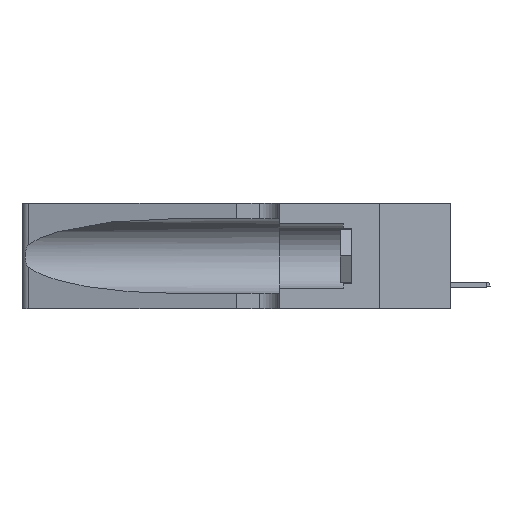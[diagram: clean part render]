
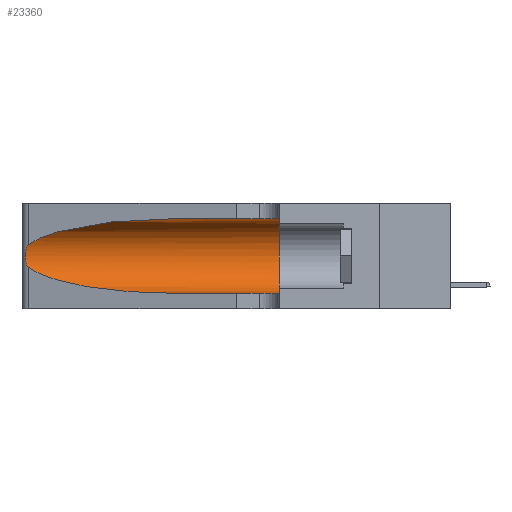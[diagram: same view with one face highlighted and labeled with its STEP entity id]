
A CAD part, left-side view. The second image highlights one B-rep face of the part: STEP entity #23360.
In plain terms, the highlighted cylindrical face has radius 3.308 mm (diameter 6.617 mm), a partial arc.
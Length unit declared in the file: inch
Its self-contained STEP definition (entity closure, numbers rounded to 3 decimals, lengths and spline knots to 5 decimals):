
#435 = ORIENTED_EDGE ( 'NONE', *, *, #18205, .T. ) ;
#545 = VERTEX_POINT ( 'NONE', #1530 ) ;
#792 = VERTEX_POINT ( 'NONE', #42409 ) ;
#1530 = CARTESIAN_POINT ( 'NONE',  ( 0.25487, 1.22718, 0.14631 ) ) ;
#2758 = VERTEX_POINT ( 'NONE', #30562 ) ;
#3268 = ORIENTED_EDGE ( 'NONE', *, *, #11400, .F. ) ;
#3404 = CARTESIAN_POINT ( 'NONE',  ( 0.25555, 1.22994, 0.2215 ) ) ;
#5291 =( BOUNDED_CURVE ( )  B_SPLINE_CURVE ( 3, ( #20249, #23532, #7633, #46288 ),
 .UNSPECIFIED., .F., .F. ) 
 B_SPLINE_CURVE_WITH_KNOTS ( ( 4, 4 ),
 ( 1.5708, 2.84003 ),
 .UNSPECIFIED. ) 
 CURVE ( )  GEOMETRIC_REPRESENTATION_ITEM ( )  RATIONAL_B_SPLINE_CURVE ( ( 1., 0.87, 0.87, 1. ) ) 
 REPRESENTATION_ITEM ( '' )  );
#5547 = DIRECTION ( 'NONE',  ( 0., -1., 0. ) ) ;
#6054 = LINE ( 'NONE', #32336, #23527 ) ;
#6379 = CARTESIAN_POINT ( 'NONE',  ( 0.2373, 1.15595, 0.08982 ) ) ;
#7177 = CARTESIAN_POINT ( 'NONE',  ( 0.25787, 1.23484, 0.2124 ) ) ;
#7300 = DIRECTION ( 'NONE',  ( 0., 1., 0. ) ) ;
#7633 = CARTESIAN_POINT ( 'NONE',  ( 0.2373, 1.15595, 0.28018 ) ) ;
#9476 = AXIS2_PLACEMENT_3D ( 'NONE', #9518, #18070, #14035 ) ;
#9518 = CARTESIAN_POINT ( 'NONE',  ( 0.1305, 1.61858, 0.185 ) ) ;
#10172 = ORIENTED_EDGE ( 'NONE', *, *, #28903, .F. ) ;
#10822 = B_SPLINE_CURVE_WITH_KNOTS ( 'NONE', 3,
 ( #15258, #3404, #15509, #7177, #14499, #22316, #26127, #14998, #33982, #49378, #14746, #18793, #19301, #22567 ),
 .UNSPECIFIED., .F., .F.,
 ( 4, 2, 2, 2, 2, 2, 4 ),
 ( 0., 0.00027, 0.00053, 0.00107, 0.0016, 0.00187, 0.00214 ),
 .UNSPECIFIED. ) ;
#11400 = EDGE_CURVE ( 'NONE', #2758, #25137, #27996, .T. ) ;
#13346 = EDGE_CURVE ( 'NONE', #792, #545, #10822, .T. ) ;
#13796 = CYLINDRICAL_SURFACE ( 'NONE', #9476, 0.13025 ) ;
#14035 = DIRECTION ( 'NONE',  ( 0., 0., -1. ) ) ;
#14499 = CARTESIAN_POINT ( 'NONE',  ( 0.25854, 1.2359, 0.20912 ) ) ;
#14746 = CARTESIAN_POINT ( 'NONE',  ( 0.25789, 1.23486, 0.15765 ) ) ;
#14998 = CARTESIAN_POINT ( 'NONE',  ( 0.26075, 1.23896, 0.178 ) ) ;
#15258 = CARTESIAN_POINT ( 'NONE',  ( 0.25487, 1.22718, 0.22369 ) ) ;
#15509 = CARTESIAN_POINT ( 'NONE',  ( 0.25639, 1.23184, 0.21858 ) ) ;
#17262 = EDGE_CURVE ( 'NONE', #39887, #47382, #6054, .T. ) ;
#18070 = DIRECTION ( 'NONE',  ( 0., -1., 0. ) ) ;
#18205 = EDGE_CURVE ( 'NONE', #545, #39887, #39839, .T. ) ;
#18793 = CARTESIAN_POINT ( 'NONE',  ( 0.25639, 1.23186, 0.15144 ) ) ;
#19301 = CARTESIAN_POINT ( 'NONE',  ( 0.25555, 1.22993, 0.14849 ) ) ;
#20249 = CARTESIAN_POINT ( 'NONE',  ( 0.1305, 0.72297, 0.31525 ) ) ;
#20498 = EDGE_CURVE ( 'NONE', #2758, #792, #5291, .T. ) ;
#21761 = CARTESIAN_POINT ( 'NONE',  ( 0.18966, 0.96281, 0.05475 ) ) ;
#22316 = CARTESIAN_POINT ( 'NONE',  ( 0.26018, 1.23835, 0.19895 ) ) ;
#22567 = CARTESIAN_POINT ( 'NONE',  ( 0.25487, 1.22718, 0.14631 ) ) ;
#23360 = ADVANCED_FACE ( 'NONE', ( #24919 ), #13796, .F. ) ;
#23527 = VECTOR ( 'NONE', #5547, 39.37008 ) ;
#23532 = CARTESIAN_POINT ( 'NONE',  ( 0.18966, 0.96281, 0.31525 ) ) ;
#24185 = CARTESIAN_POINT ( 'NONE',  ( 0.1305, 1.61858, 0.31525 ) ) ;
#24919 = FACE_OUTER_BOUND ( 'NONE', #25611, .T. ) ;
#25137 = VERTEX_POINT ( 'NONE', #34955 ) ;
#25611 = EDGE_LOOP ( 'NONE', ( #44014, #34714, #435, #33272, #10172, #3268 ) ) ;
#26127 = CARTESIAN_POINT ( 'NONE',  ( 0.26075, 1.23896, 0.19203 ) ) ;
#27996 = LINE ( 'NONE', #24185, #48833 ) ;
#28903 = EDGE_CURVE ( 'NONE', #25137, #47382, #45477, .T. ) ;
#30562 = CARTESIAN_POINT ( 'NONE',  ( 0.1305, 0.72297, 0.31525 ) ) ;
#32336 = CARTESIAN_POINT ( 'NONE',  ( 0.1305, 1.61858, 0.05475 ) ) ;
#33272 = ORIENTED_EDGE ( 'NONE', *, *, #17262, .T. ) ;
#33982 = CARTESIAN_POINT ( 'NONE',  ( 0.26017, 1.23833, 0.17102 ) ) ;
#34714 = ORIENTED_EDGE ( 'NONE', *, *, #13346, .T. ) ;
#34955 = CARTESIAN_POINT ( 'NONE',  ( 0.1305, 0.35, 0.31525 ) ) ;
#35733 = CARTESIAN_POINT ( 'NONE',  ( 0.1305, 0.72297, 0.05475 ) ) ;
#37210 = CARTESIAN_POINT ( 'NONE',  ( 0.1305, 0.72297, 0.05475 ) ) ;
#39622 = DIRECTION ( 'NONE',  ( 0., -1., 0. ) ) ;
#39839 =( BOUNDED_CURVE ( )  B_SPLINE_CURVE ( 3, ( #40999, #6379, #21761, #37210 ),
 .UNSPECIFIED., .F., .F. ) 
 B_SPLINE_CURVE_WITH_KNOTS ( ( 4, 4 ),
 ( 3.44316, 4.71239 ),
 .UNSPECIFIED. ) 
 CURVE ( )  GEOMETRIC_REPRESENTATION_ITEM ( )  RATIONAL_B_SPLINE_CURVE ( ( 1., 0.87, 0.87, 1. ) ) 
 REPRESENTATION_ITEM ( '' )  );
#39887 = VERTEX_POINT ( 'NONE', #35733 ) ;
#40999 = CARTESIAN_POINT ( 'NONE',  ( 0.25487, 1.22718, 0.14631 ) ) ;
#42409 = CARTESIAN_POINT ( 'NONE',  ( 0.25487, 1.22718, 0.22369 ) ) ;
#42418 = DIRECTION ( 'NONE',  ( 0., 0., 1. ) ) ;
#43868 = AXIS2_PLACEMENT_3D ( 'NONE', #46204, #7300, #42418 ) ;
#44014 = ORIENTED_EDGE ( 'NONE', *, *, #20498, .T. ) ;
#45477 = CIRCLE ( 'NONE', #43868, 0.13025 ) ;
#45797 = CARTESIAN_POINT ( 'NONE',  ( 0.1305, 0.35, 0.05475 ) ) ;
#46204 = CARTESIAN_POINT ( 'NONE',  ( 0.1305, 0.35, 0.185 ) ) ;
#46288 = CARTESIAN_POINT ( 'NONE',  ( 0.25487, 1.22718, 0.22369 ) ) ;
#47382 = VERTEX_POINT ( 'NONE', #45797 ) ;
#48833 = VECTOR ( 'NONE', #39622, 39.37008 ) ;
#49378 = CARTESIAN_POINT ( 'NONE',  ( 0.25856, 1.23593, 0.16098 ) ) ;
